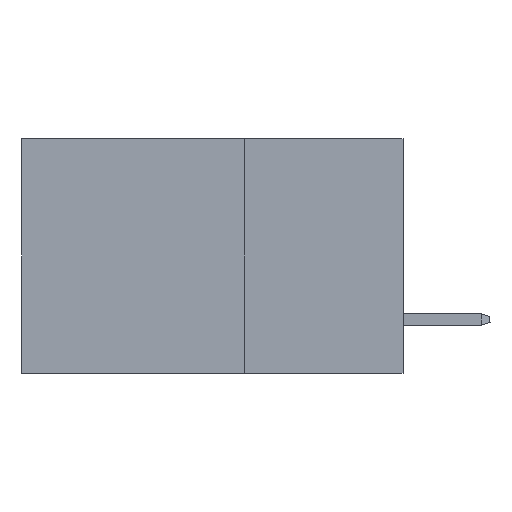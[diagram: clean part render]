
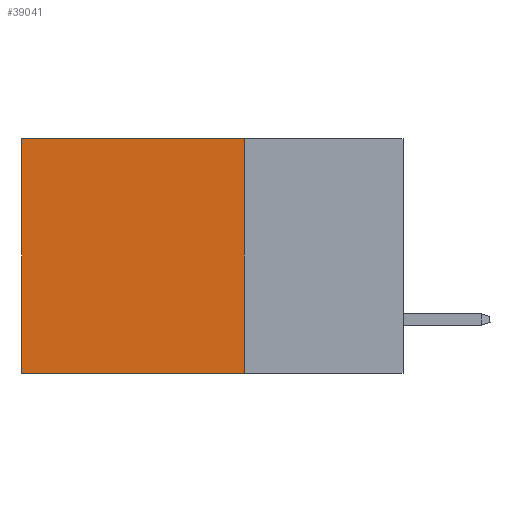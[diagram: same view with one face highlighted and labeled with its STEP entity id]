
A CAD part, left-side view. The second image highlights one B-rep face of the part: STEP entity #39041.
In plain terms, the highlighted planar face has unit normal (-1, 0, 0).
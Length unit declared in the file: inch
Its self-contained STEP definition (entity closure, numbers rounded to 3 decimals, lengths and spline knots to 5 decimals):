
#218 = CARTESIAN_POINT ( 'NONE',  ( 0.2875, 0.25, -0.37 ) ) ;
#3327 = LINE ( 'NONE', #218, #32554 ) ;
#6315 = CARTESIAN_POINT ( 'NONE',  ( 0.2875, 0.6, -0.37 ) ) ;
#6407 = CARTESIAN_POINT ( 'NONE',  ( 0.2875, 0.25, 0. ) ) ;
#9446 = VECTOR ( 'NONE', #32491, 39.37008 ) ;
#10289 = EDGE_CURVE ( 'NONE', #32766, #19565, #30148, .T. ) ;
#10417 = CARTESIAN_POINT ( 'NONE',  ( 0.2875, 0.25, 0. ) ) ;
#17401 = EDGE_CURVE ( 'NONE', #32766, #31178, #23079, .T. ) ;
#17563 = ORIENTED_EDGE ( 'NONE', *, *, #10289, .F. ) ;
#18658 = PLANE ( 'NONE',  #29005 ) ;
#19120 = ORIENTED_EDGE ( 'NONE', *, *, #23996, .T. ) ;
#19565 = VERTEX_POINT ( 'NONE', #39150 ) ;
#21791 = FACE_OUTER_BOUND ( 'NONE', #36969, .T. ) ;
#22195 = DIRECTION ( 'NONE',  ( 1., 0., 0. ) ) ;
#22439 = VERTEX_POINT ( 'NONE', #6315 ) ;
#22768 = DIRECTION ( 'NONE',  ( 0., 1., 0. ) ) ;
#22808 = EDGE_CURVE ( 'NONE', #19565, #22439, #3327, .T. ) ;
#23079 = LINE ( 'NONE', #10417, #38287 ) ;
#23167 = LINE ( 'NONE', #29205, #9446 ) ;
#23922 = DIRECTION ( 'NONE',  ( 0., 0., -1. ) ) ;
#23996 = EDGE_CURVE ( 'NONE', #31178, #22439, #23167, .T. ) ;
#24898 = CARTESIAN_POINT ( 'NONE',  ( 0.2875, 0.25, 0. ) ) ;
#28062 = ORIENTED_EDGE ( 'NONE', *, *, #17401, .T. ) ;
#28838 = DIRECTION ( 'NONE',  ( 0., 0., -1. ) ) ;
#28839 = VECTOR ( 'NONE', #23922, 39.37008 ) ;
#29005 = AXIS2_PLACEMENT_3D ( 'NONE', #24898, #22195, #28838 ) ;
#29205 = CARTESIAN_POINT ( 'NONE',  ( 0.2875, 0.6, 0. ) ) ;
#30148 = LINE ( 'NONE', #39680, #28839 ) ;
#30191 = ORIENTED_EDGE ( 'NONE', *, *, #22808, .F. ) ;
#31178 = VERTEX_POINT ( 'NONE', #35393 ) ;
#32491 = DIRECTION ( 'NONE',  ( 0., 0., -1. ) ) ;
#32554 = VECTOR ( 'NONE', #22768, 39.37008 ) ;
#32766 = VERTEX_POINT ( 'NONE', #6407 ) ;
#35110 = DIRECTION ( 'NONE',  ( 0., 1., 0. ) ) ;
#35393 = CARTESIAN_POINT ( 'NONE',  ( 0.2875, 0.6, 0. ) ) ;
#36969 = EDGE_LOOP ( 'NONE', ( #19120, #30191, #17563, #28062 ) ) ;
#38287 = VECTOR ( 'NONE', #35110, 39.37008 ) ;
#39041 = ADVANCED_FACE ( 'NONE', ( #21791 ), #18658, .F. ) ;
#39150 = CARTESIAN_POINT ( 'NONE',  ( 0.2875, 0.25, -0.37 ) ) ;
#39680 = CARTESIAN_POINT ( 'NONE',  ( 0.2875, 0.25, 0. ) ) ;
